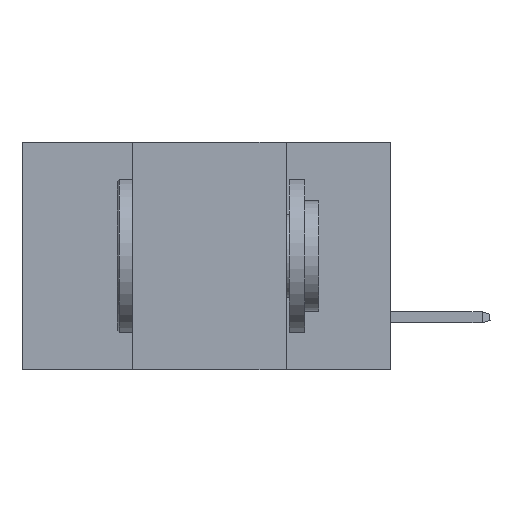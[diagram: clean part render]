
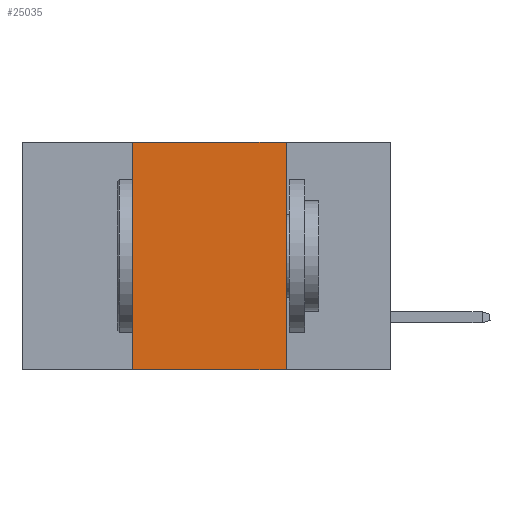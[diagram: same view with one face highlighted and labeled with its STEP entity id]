
A CAD part, left-side view. The second image highlights one B-rep face of the part: STEP entity #25035.
In plain terms, the highlighted planar face has unit normal (-1, 0, 0).
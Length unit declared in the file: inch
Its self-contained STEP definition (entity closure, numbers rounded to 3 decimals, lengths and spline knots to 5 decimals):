
#1686 = ORIENTED_EDGE ( 'NONE', *, *, #14556, .F. ) ;
#1788 = CARTESIAN_POINT ( 'NONE',  ( 0., 0.6, 0. ) ) ;
#3209 = LINE ( 'NONE', #24113, #25540 ) ;
#3380 = DIRECTION ( 'NONE',  ( 0., -1., 0. ) ) ;
#4939 = VECTOR ( 'NONE', #35538, 39.37008 ) ;
#5822 = LINE ( 'NONE', #32578, #4939 ) ;
#7061 = VERTEX_POINT ( 'NONE', #7154 ) ;
#7154 = CARTESIAN_POINT ( 'NONE',  ( 0., 0.17, -0.37 ) ) ;
#7794 = DIRECTION ( 'NONE',  ( 1., 0., 0. ) ) ;
#9080 = EDGE_CURVE ( 'NONE', #13944, #16490, #3209, .T. ) ;
#9621 = VECTOR ( 'NONE', #25511, 39.37008 ) ;
#12098 = VERTEX_POINT ( 'NONE', #34621 ) ;
#12907 = AXIS2_PLACEMENT_3D ( 'NONE', #1788, #7794, #35599 ) ;
#13284 = DIRECTION ( 'NONE',  ( 0., 0., 1. ) ) ;
#13944 = VERTEX_POINT ( 'NONE', #33625 ) ;
#14556 = EDGE_CURVE ( 'NONE', #12098, #7061, #27884, .T. ) ;
#14559 = EDGE_LOOP ( 'NONE', ( #1686, #30218, #34194, #29945 ) ) ;
#16490 = VERTEX_POINT ( 'NONE', #16582 ) ;
#16582 = CARTESIAN_POINT ( 'NONE',  ( 0., 0.42, 0. ) ) ;
#17625 = FACE_OUTER_BOUND ( 'NONE', #14559, .T. ) ;
#18563 = VECTOR ( 'NONE', #3380, 39.37008 ) ;
#21991 = PLANE ( 'NONE',  #12907 ) ;
#24113 = CARTESIAN_POINT ( 'NONE',  ( 0., 0.42, 0. ) ) ;
#25035 = ADVANCED_FACE ( 'NONE', ( #17625 ), #21991, .F. ) ;
#25511 = DIRECTION ( 'NONE',  ( 0., 0., -1. ) ) ;
#25540 = VECTOR ( 'NONE', #13284, 39.37008 ) ;
#27884 = LINE ( 'NONE', #30346, #9621 ) ;
#28135 = EDGE_CURVE ( 'NONE', #13944, #7061, #35401, .T. ) ;
#29945 = ORIENTED_EDGE ( 'NONE', *, *, #28135, .T. ) ;
#30218 = ORIENTED_EDGE ( 'NONE', *, *, #34075, .F. ) ;
#30346 = CARTESIAN_POINT ( 'NONE',  ( 0., 0.17, 0. ) ) ;
#31617 = CARTESIAN_POINT ( 'NONE',  ( 0., 0.6, -0.37 ) ) ;
#32578 = CARTESIAN_POINT ( 'NONE',  ( 0., 0.6, 0. ) ) ;
#33625 = CARTESIAN_POINT ( 'NONE',  ( 0., 0.42, -0.37 ) ) ;
#34075 = EDGE_CURVE ( 'NONE', #16490, #12098, #5822, .T. ) ;
#34194 = ORIENTED_EDGE ( 'NONE', *, *, #9080, .F. ) ;
#34621 = CARTESIAN_POINT ( 'NONE',  ( 0., 0.17, 0. ) ) ;
#35401 = LINE ( 'NONE', #31617, #18563 ) ;
#35538 = DIRECTION ( 'NONE',  ( 0., -1., 0. ) ) ;
#35599 = DIRECTION ( 'NONE',  ( 0., 0., -1. ) ) ;
